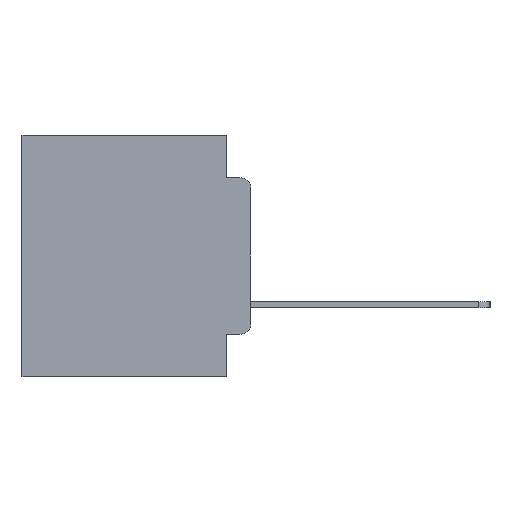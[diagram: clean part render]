
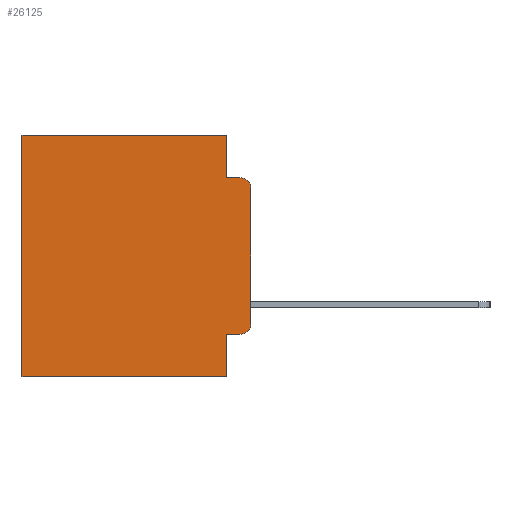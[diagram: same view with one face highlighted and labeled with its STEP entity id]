
A CAD part, left-side view. The second image highlights one B-rep face of the part: STEP entity #26125.
In plain terms, the highlighted planar face has unit normal (-1, 0, 0).
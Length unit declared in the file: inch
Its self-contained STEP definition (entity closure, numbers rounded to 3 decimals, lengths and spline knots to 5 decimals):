
#221 = EDGE_CURVE ( 'NONE', #361, #21008, #1155, .T. ) ;
#361 = VERTEX_POINT ( 'NONE', #1871 ) ;
#650 = LINE ( 'NONE', #27223, #28913 ) ;
#1155 = LINE ( 'NONE', #12366, #12719 ) ;
#1740 = DIRECTION ( 'NONE',  ( 1., 0., 0. ) ) ;
#1871 = CARTESIAN_POINT ( 'NONE',  ( 0.298, 0.051, -0.5 ) ) ;
#2084 = CARTESIAN_POINT ( 'NONE',  ( 0.298, 0.051, 0. ) ) ;
#2087 = VECTOR ( 'NONE', #5902, 39.37008 ) ;
#2814 = LINE ( 'NONE', #19951, #2087 ) ;
#3133 = EDGE_CURVE ( 'NONE', #16435, #7659, #2814, .T. ) ;
#3518 = CARTESIAN_POINT ( 'NONE',  ( 0.298, 0.02, -0.1085 ) ) ;
#3694 = VECTOR ( 'NONE', #11089, 39.37008 ) ;
#5259 = EDGE_CURVE ( 'NONE', #7510, #21008, #24962, .T. ) ;
#5870 = DIRECTION ( 'NONE',  ( 0., 0., -1. ) ) ;
#5902 = DIRECTION ( 'NONE',  ( 0., -1., 0. ) ) ;
#6259 = AXIS2_PLACEMENT_3D ( 'NONE', #3518, #19494, #5870 ) ;
#6530 = CARTESIAN_POINT ( 'NONE',  ( 0.298, 0.051, 0. ) ) ;
#6561 = AXIS2_PLACEMENT_3D ( 'NONE', #25755, #12597, #27855 ) ;
#6740 = DIRECTION ( 'NONE',  ( 0., 0., -1. ) ) ;
#6836 = EDGE_CURVE ( 'NONE', #21319, #23117, #8103, .T. ) ;
#7510 = VERTEX_POINT ( 'NONE', #21616 ) ;
#7547 = CARTESIAN_POINT ( 'NONE',  ( 0.298, 0.051, -0.0885 ) ) ;
#7659 = VERTEX_POINT ( 'NONE', #8619 ) ;
#7716 = ORIENTED_EDGE ( 'NONE', *, *, #221, .F. ) ;
#8062 = ORIENTED_EDGE ( 'NONE', *, *, #24723, .T. ) ;
#8103 = CIRCLE ( 'NONE', #6561, 0.02 ) ;
#8619 = CARTESIAN_POINT ( 'NONE',  ( 0.298, 0.02, -0.0885 ) ) ;
#9166 = LINE ( 'NONE', #15637, #3694 ) ;
#9911 = ORIENTED_EDGE ( 'NONE', *, *, #3133, .F. ) ;
#10131 = LINE ( 'NONE', #12669, #16123 ) ;
#10925 = CARTESIAN_POINT ( 'NONE',  ( 0.298, 0.051, -0.4115 ) ) ;
#10952 = PLANE ( 'NONE',  #15710 ) ;
#11089 = DIRECTION ( 'NONE',  ( 0., 0., -1. ) ) ;
#11126 = DIRECTION ( 'NONE',  ( 0., 0., -1. ) ) ;
#11148 = CIRCLE ( 'NONE', #6259, 0.02 ) ;
#11541 = LINE ( 'NONE', #25559, #16835 ) ;
#12138 = VERTEX_POINT ( 'NONE', #6530 ) ;
#12366 = CARTESIAN_POINT ( 'NONE',  ( 0.298, 0., -0.5 ) ) ;
#12597 = DIRECTION ( 'NONE',  ( -1., 0., 0. ) ) ;
#12669 = CARTESIAN_POINT ( 'NONE',  ( 0.298, 0., 0. ) ) ;
#12719 = VECTOR ( 'NONE', #15010, 39.37008 ) ;
#13233 = CARTESIAN_POINT ( 'NONE',  ( 0.298, 0., 0. ) ) ;
#13237 = VECTOR ( 'NONE', #11126, 39.37008 ) ;
#14953 = CARTESIAN_POINT ( 'NONE',  ( 0.298, 0.473, -0.5 ) ) ;
#15010 = DIRECTION ( 'NONE',  ( 0., 1., 0. ) ) ;
#15252 = CARTESIAN_POINT ( 'NONE',  ( 0.298, 0.473, 0. ) ) ;
#15637 = CARTESIAN_POINT ( 'NONE',  ( 0.298, 0., 0. ) ) ;
#15710 = AXIS2_PLACEMENT_3D ( 'NONE', #13233, #1740, #17757 ) ;
#16123 = VECTOR ( 'NONE', #27928, 39.37008 ) ;
#16435 = VERTEX_POINT ( 'NONE', #7547 ) ;
#16534 = DIRECTION ( 'NONE',  ( 0., -1., 0. ) ) ;
#16768 = EDGE_CURVE ( 'NONE', #21256, #23117, #9166, .T. ) ;
#16835 = VECTOR ( 'NONE', #23513, 39.37008 ) ;
#17327 = ORIENTED_EDGE ( 'NONE', *, *, #21234, .F. ) ;
#17350 = ORIENTED_EDGE ( 'NONE', *, *, #24679, .F. ) ;
#17757 = DIRECTION ( 'NONE',  ( 0., 0., -1. ) ) ;
#17876 = LINE ( 'NONE', #2084, #23669 ) ;
#18460 = FACE_OUTER_BOUND ( 'NONE', #21553, .T. ) ;
#19494 = DIRECTION ( 'NONE',  ( -1., 0., 0. ) ) ;
#19951 = CARTESIAN_POINT ( 'NONE',  ( 0.298, 0.051, -0.0885 ) ) ;
#20027 = VERTEX_POINT ( 'NONE', #10925 ) ;
#20146 = CARTESIAN_POINT ( 'NONE',  ( 0.298, 0., -0.3915 ) ) ;
#21008 = VERTEX_POINT ( 'NONE', #14953 ) ;
#21234 = EDGE_CURVE ( 'NONE', #12138, #16435, #17876, .T. ) ;
#21256 = VERTEX_POINT ( 'NONE', #28862 ) ;
#21319 = VERTEX_POINT ( 'NONE', #26945 ) ;
#21403 = EDGE_CURVE ( 'NONE', #20027, #21319, #650, .T. ) ;
#21493 = ORIENTED_EDGE ( 'NONE', *, *, #5259, .T. ) ;
#21553 = EDGE_LOOP ( 'NONE', ( #28024, #23474, #9911, #17327, #8062, #21493, #7716, #17350, #23842, #22189 ) ) ;
#21616 = CARTESIAN_POINT ( 'NONE',  ( 0.298, 0.473, 0. ) ) ;
#22189 = ORIENTED_EDGE ( 'NONE', *, *, #6836, .T. ) ;
#23117 = VERTEX_POINT ( 'NONE', #20146 ) ;
#23474 = ORIENTED_EDGE ( 'NONE', *, *, #25374, .T. ) ;
#23513 = DIRECTION ( 'NONE',  ( 0., 0., -1. ) ) ;
#23669 = VECTOR ( 'NONE', #6740, 39.37008 ) ;
#23842 = ORIENTED_EDGE ( 'NONE', *, *, #21403, .T. ) ;
#24679 = EDGE_CURVE ( 'NONE', #20027, #361, #11541, .T. ) ;
#24723 = EDGE_CURVE ( 'NONE', #12138, #7510, #10131, .T. ) ;
#24962 = LINE ( 'NONE', #15252, #13237 ) ;
#25374 = EDGE_CURVE ( 'NONE', #21256, #7659, #11148, .T. ) ;
#25559 = CARTESIAN_POINT ( 'NONE',  ( 0.298, 0.051, 0. ) ) ;
#25755 = CARTESIAN_POINT ( 'NONE',  ( 0.298, 0.02, -0.3915 ) ) ;
#26125 = ADVANCED_FACE ( 'NONE', ( #18460 ), #10952, .F. ) ;
#26945 = CARTESIAN_POINT ( 'NONE',  ( 0.298, 0.02, -0.4115 ) ) ;
#27223 = CARTESIAN_POINT ( 'NONE',  ( 0.298, 0.051, -0.4115 ) ) ;
#27855 = DIRECTION ( 'NONE',  ( 0., 0., -1. ) ) ;
#27928 = DIRECTION ( 'NONE',  ( 0., 1., 0. ) ) ;
#28024 = ORIENTED_EDGE ( 'NONE', *, *, #16768, .F. ) ;
#28862 = CARTESIAN_POINT ( 'NONE',  ( 0.298, 0., -0.1085 ) ) ;
#28913 = VECTOR ( 'NONE', #16534, 39.37008 ) ;
